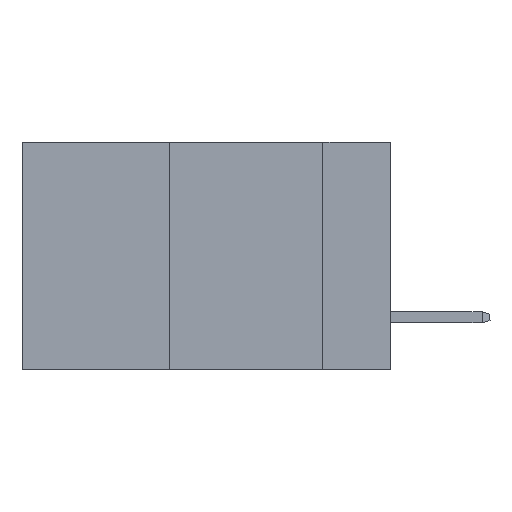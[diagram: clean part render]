
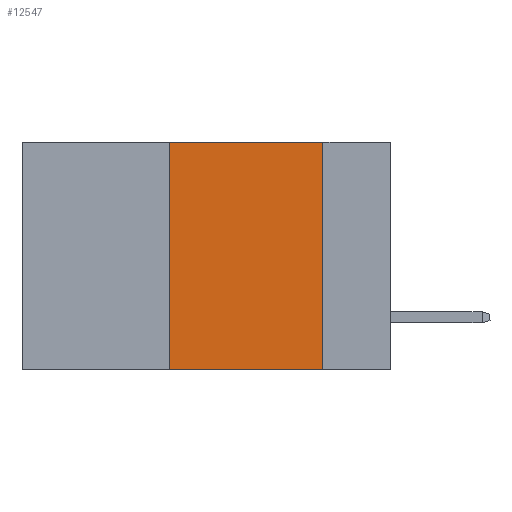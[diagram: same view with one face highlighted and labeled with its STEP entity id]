
A CAD part, left-side view. The second image highlights one B-rep face of the part: STEP entity #12547.
In plain terms, the highlighted planar face has unit normal (-1, 0, 0).
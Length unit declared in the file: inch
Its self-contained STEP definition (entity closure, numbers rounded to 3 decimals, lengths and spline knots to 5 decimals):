
#284 = CARTESIAN_POINT ( 'NONE',  ( 0., 0.11, 0. ) ) ;
#533 = PLANE ( 'NONE',  #5517 ) ;
#641 = CARTESIAN_POINT ( 'NONE',  ( 0., 0.11, 0. ) ) ;
#823 = LINE ( 'NONE', #3238, #10759 ) ;
#1182 = EDGE_CURVE ( 'NONE', #13934, #10235, #9574, .T. ) ;
#2013 = VERTEX_POINT ( 'NONE', #9025 ) ;
#2888 = VECTOR ( 'NONE', #13671, 39.37008 ) ;
#2900 = CARTESIAN_POINT ( 'NONE',  ( 0., 0.36, -0.37 ) ) ;
#3018 = DIRECTION ( 'NONE',  ( 0., 0., -1. ) ) ;
#3238 = CARTESIAN_POINT ( 'NONE',  ( 0., 0.6, 0. ) ) ;
#3648 = EDGE_CURVE ( 'NONE', #6602, #2013, #8534, .T. ) ;
#3926 = FACE_OUTER_BOUND ( 'NONE', #9456, .T. ) ;
#4506 = DIRECTION ( 'NONE',  ( 0., -1., 0. ) ) ;
#4579 = ORIENTED_EDGE ( 'NONE', *, *, #1182, .F. ) ;
#5517 = AXIS2_PLACEMENT_3D ( 'NONE', #9305, #10505, #3018 ) ;
#5654 = CARTESIAN_POINT ( 'NONE',  ( 0., 0.6, -0.37 ) ) ;
#6199 = EDGE_CURVE ( 'NONE', #6602, #10235, #6343, .T. ) ;
#6343 = LINE ( 'NONE', #5654, #12809 ) ;
#6602 = VERTEX_POINT ( 'NONE', #2900 ) ;
#7482 = EDGE_CURVE ( 'NONE', #2013, #13934, #823, .T. ) ;
#8534 = LINE ( 'NONE', #12886, #11706 ) ;
#8664 = ORIENTED_EDGE ( 'NONE', *, *, #6199, .T. ) ;
#9025 = CARTESIAN_POINT ( 'NONE',  ( 0., 0.36, 0. ) ) ;
#9305 = CARTESIAN_POINT ( 'NONE',  ( 0., 0.6, 0. ) ) ;
#9453 = DIRECTION ( 'NONE',  ( 0., -1., 0. ) ) ;
#9456 = EDGE_LOOP ( 'NONE', ( #4579, #11341, #14016, #8664 ) ) ;
#9574 = LINE ( 'NONE', #284, #2888 ) ;
#10235 = VERTEX_POINT ( 'NONE', #11254 ) ;
#10505 = DIRECTION ( 'NONE',  ( 1., 0., 0. ) ) ;
#10759 = VECTOR ( 'NONE', #4506, 39.37008 ) ;
#11254 = CARTESIAN_POINT ( 'NONE',  ( 0., 0.11, -0.37 ) ) ;
#11341 = ORIENTED_EDGE ( 'NONE', *, *, #7482, .F. ) ;
#11706 = VECTOR ( 'NONE', #12974, 39.37008 ) ;
#12547 = ADVANCED_FACE ( 'NONE', ( #3926 ), #533, .F. ) ;
#12809 = VECTOR ( 'NONE', #9453, 39.37008 ) ;
#12886 = CARTESIAN_POINT ( 'NONE',  ( 0., 0.36, 0. ) ) ;
#12974 = DIRECTION ( 'NONE',  ( 0., 0., 1. ) ) ;
#13671 = DIRECTION ( 'NONE',  ( 0., 0., -1. ) ) ;
#13934 = VERTEX_POINT ( 'NONE', #641 ) ;
#14016 = ORIENTED_EDGE ( 'NONE', *, *, #3648, .F. ) ;
